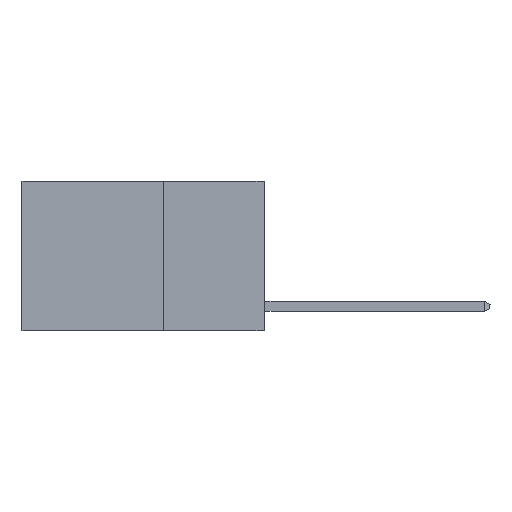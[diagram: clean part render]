
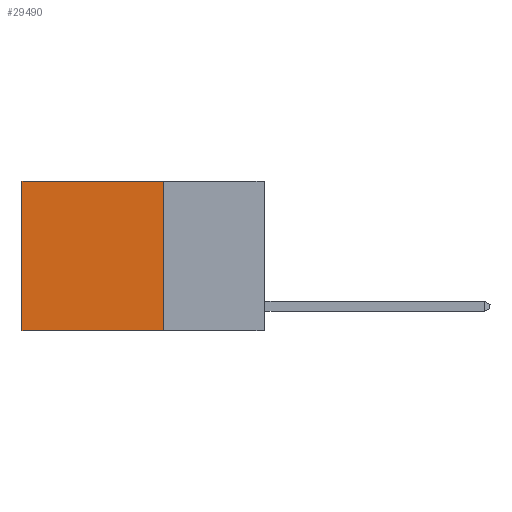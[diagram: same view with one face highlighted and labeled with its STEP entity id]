
A CAD part, left-side view. The second image highlights one B-rep face of the part: STEP entity #29490.
In plain terms, the highlighted planar face has unit normal (-1, 0, 0).
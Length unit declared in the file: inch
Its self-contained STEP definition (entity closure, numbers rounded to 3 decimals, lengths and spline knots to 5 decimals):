
#233 = EDGE_CURVE ( 'NONE', #11857, #25984, #29501, .T. ) ;
#903 = VERTEX_POINT ( 'NONE', #10536 ) ;
#3365 = PLANE ( 'NONE',  #19927 ) ;
#3888 = ORIENTED_EDGE ( 'NONE', *, *, #21790, .F. ) ;
#3960 = EDGE_LOOP ( 'NONE', ( #19559, #28634, #3888, #5926 ) ) ;
#5047 = CARTESIAN_POINT ( 'NONE',  ( 0.2625, 0.6, 0. ) ) ;
#5926 = ORIENTED_EDGE ( 'NONE', *, *, #26542, .T. ) ;
#7364 = CARTESIAN_POINT ( 'NONE',  ( 0.2625, 0.25, 0. ) ) ;
#7471 = DIRECTION ( 'NONE',  ( 0., 0., -1. ) ) ;
#8369 = CARTESIAN_POINT ( 'NONE',  ( 0.2625, 0.25, 0. ) ) ;
#8944 = VERTEX_POINT ( 'NONE', #26422 ) ;
#9140 = VECTOR ( 'NONE', #24830, 39.37008 ) ;
#9199 = VECTOR ( 'NONE', #26382, 39.37008 ) ;
#9788 = LINE ( 'NONE', #7364, #28253 ) ;
#9925 = DIRECTION ( 'NONE',  ( 1., 0., 0. ) ) ;
#10536 = CARTESIAN_POINT ( 'NONE',  ( 0.2625, 0.6, 0. ) ) ;
#10643 = LINE ( 'NONE', #8369, #9199 ) ;
#11857 = VERTEX_POINT ( 'NONE', #28377 ) ;
#12334 = CARTESIAN_POINT ( 'NONE',  ( 0.2625, 0.25, 0. ) ) ;
#13045 = VECTOR ( 'NONE', #7471, 39.37008 ) ;
#13491 = CARTESIAN_POINT ( 'NONE',  ( 0.2625, 0.25, -0.37 ) ) ;
#13971 = LINE ( 'NONE', #5047, #13045 ) ;
#14413 = CARTESIAN_POINT ( 'NONE',  ( 0.2625, 0.6, -0.37 ) ) ;
#16602 = DIRECTION ( 'NONE',  ( 0., 0., -1. ) ) ;
#16877 = DIRECTION ( 'NONE',  ( 0., 0., -1. ) ) ;
#19559 = ORIENTED_EDGE ( 'NONE', *, *, #25863, .T. ) ;
#19927 = AXIS2_PLACEMENT_3D ( 'NONE', #12334, #9925, #16877 ) ;
#21790 = EDGE_CURVE ( 'NONE', #8944, #11857, #9788, .T. ) ;
#24830 = DIRECTION ( 'NONE',  ( 0., 1., 0. ) ) ;
#25863 = EDGE_CURVE ( 'NONE', #903, #25984, #13971, .T. ) ;
#25984 = VERTEX_POINT ( 'NONE', #14413 ) ;
#26382 = DIRECTION ( 'NONE',  ( 0., 1., 0. ) ) ;
#26422 = CARTESIAN_POINT ( 'NONE',  ( 0.2625, 0.25, 0. ) ) ;
#26542 = EDGE_CURVE ( 'NONE', #8944, #903, #10643, .T. ) ;
#28253 = VECTOR ( 'NONE', #16602, 39.37008 ) ;
#28377 = CARTESIAN_POINT ( 'NONE',  ( 0.2625, 0.25, -0.37 ) ) ;
#28634 = ORIENTED_EDGE ( 'NONE', *, *, #233, .F. ) ;
#28926 = FACE_OUTER_BOUND ( 'NONE', #3960, .T. ) ;
#29490 = ADVANCED_FACE ( 'NONE', ( #28926 ), #3365, .F. ) ;
#29501 = LINE ( 'NONE', #13491, #9140 ) ;
